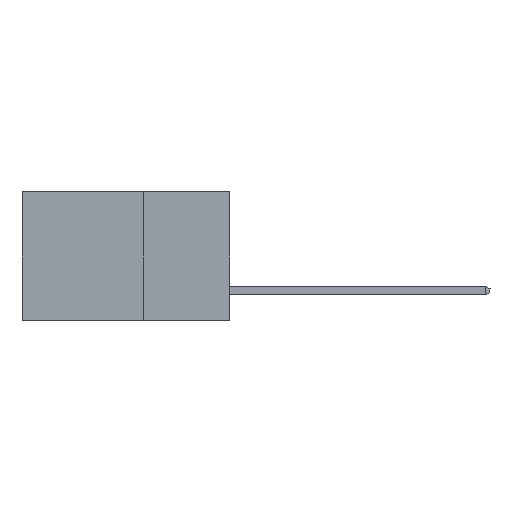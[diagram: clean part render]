
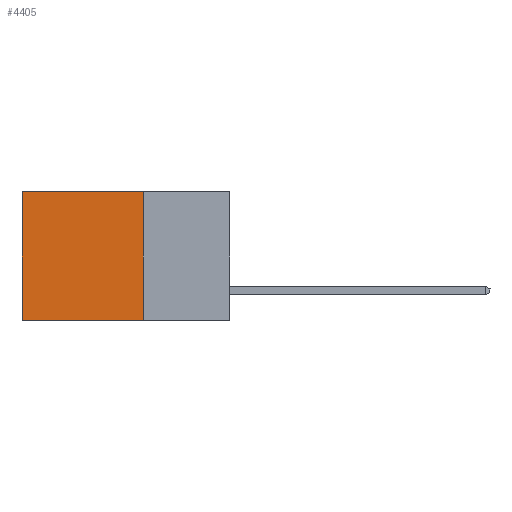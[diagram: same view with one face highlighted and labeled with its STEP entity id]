
A CAD part, left-side view. The second image highlights one B-rep face of the part: STEP entity #4405.
In plain terms, the highlighted planar face has unit normal (-1, 0, 0).
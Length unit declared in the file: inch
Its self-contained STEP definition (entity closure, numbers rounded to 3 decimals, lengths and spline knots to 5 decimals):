
#4 = CARTESIAN_POINT ( 'NONE',  ( 0.2615, 0.25, 0. ) ) ;
#87 = CARTESIAN_POINT ( 'NONE',  ( 0.2615, 0.25, -0.37 ) ) ;
#107 = VERTEX_POINT ( 'NONE', #4 ) ;
#195 = ORIENTED_EDGE ( 'NONE', *, *, #692, .F. ) ;
#573 = VERTEX_POINT ( 'NONE', #2426 ) ;
#692 = EDGE_CURVE ( 'NONE', #107, #3293, #11933, .T. ) ;
#1410 = EDGE_CURVE ( 'NONE', #3293, #4800, #10393, .T. ) ;
#1576 = DIRECTION ( 'NONE',  ( 0., 0., -1. ) ) ;
#2159 = DIRECTION ( 'NONE',  ( 0., 0., -1. ) ) ;
#2426 = CARTESIAN_POINT ( 'NONE',  ( 0.2615, 0.6, 0. ) ) ;
#3293 = VERTEX_POINT ( 'NONE', #13663 ) ;
#3719 = DIRECTION ( 'NONE',  ( 0., 1., 0. ) ) ;
#3829 = CARTESIAN_POINT ( 'NONE',  ( 0.2615, 0.25, -0.37 ) ) ;
#3937 = CARTESIAN_POINT ( 'NONE',  ( 0.2615, 0.6, -0.37 ) ) ;
#4045 = CARTESIAN_POINT ( 'NONE',  ( 0.2615, 0.6, -0.37 ) ) ;
#4046 = ORIENTED_EDGE ( 'NONE', *, *, #10823, .T. ) ;
#4405 = ADVANCED_FACE ( 'NONE', ( #10846 ), #7245, .F. ) ;
#4697 = CARTESIAN_POINT ( 'NONE',  ( 0.2615, 0.25, 0. ) ) ;
#4800 = VERTEX_POINT ( 'NONE', #3937 ) ;
#5077 = DIRECTION ( 'NONE',  ( 1., 0., 0. ) ) ;
#5602 = EDGE_LOOP ( 'NONE', ( #5823, #10771, #195, #4046 ) ) ;
#5606 = LINE ( 'NONE', #4045, #8558 ) ;
#5667 = AXIS2_PLACEMENT_3D ( 'NONE', #8520, #5077, #6355 ) ;
#5823 = ORIENTED_EDGE ( 'NONE', *, *, #5902, .T. ) ;
#5824 = VECTOR ( 'NONE', #9198, 39.37008 ) ;
#5902 = EDGE_CURVE ( 'NONE', #573, #4800, #5606, .T. ) ;
#6355 = DIRECTION ( 'NONE',  ( 0., 0., -1. ) ) ;
#6463 = VECTOR ( 'NONE', #1576, 39.37008 ) ;
#7245 = PLANE ( 'NONE',  #5667 ) ;
#8520 = CARTESIAN_POINT ( 'NONE',  ( 0.2615, 0.25, -0.37 ) ) ;
#8558 = VECTOR ( 'NONE', #2159, 39.37008 ) ;
#9198 = DIRECTION ( 'NONE',  ( 0., 1., 0. ) ) ;
#9460 = LINE ( 'NONE', #4697, #12970 ) ;
#10393 = LINE ( 'NONE', #87, #5824 ) ;
#10771 = ORIENTED_EDGE ( 'NONE', *, *, #1410, .F. ) ;
#10823 = EDGE_CURVE ( 'NONE', #107, #573, #9460, .T. ) ;
#10846 = FACE_OUTER_BOUND ( 'NONE', #5602, .T. ) ;
#11933 = LINE ( 'NONE', #3829, #6463 ) ;
#12970 = VECTOR ( 'NONE', #3719, 39.37008 ) ;
#13663 = CARTESIAN_POINT ( 'NONE',  ( 0.2615, 0.25, -0.37 ) ) ;
